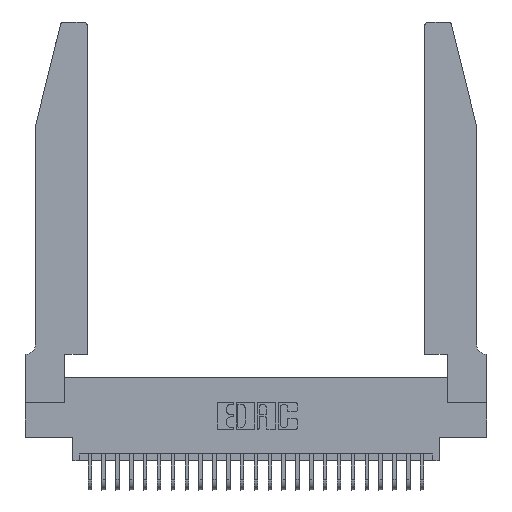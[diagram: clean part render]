
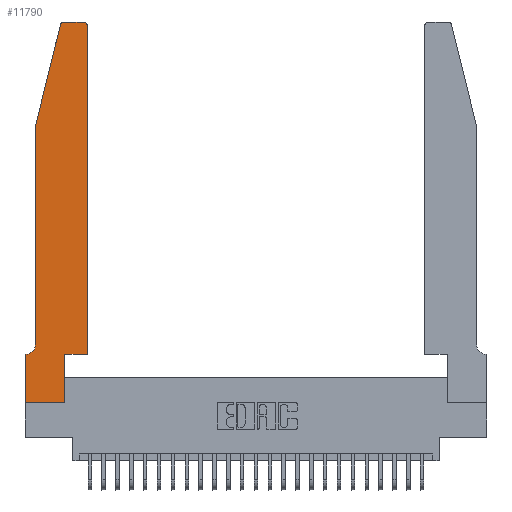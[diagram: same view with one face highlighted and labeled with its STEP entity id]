
A CAD part, top view. The second image highlights one B-rep face of the part: STEP entity #11790.
In plain terms, the highlighted planar face has unit normal (0, 0, 1).
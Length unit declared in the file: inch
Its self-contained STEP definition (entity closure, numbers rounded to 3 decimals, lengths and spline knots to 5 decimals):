
#245 = LINE ( 'NONE', #523, #20498 ) ;
#523 = CARTESIAN_POINT ( 'NONE',  ( 0.0755, 0.35, 0.37 ) ) ;
#1278 = ORIENTED_EDGE ( 'NONE', *, *, #17317, .T. ) ;
#1521 = AXIS2_PLACEMENT_3D ( 'NONE', #6994, #6895, #2677 ) ;
#1641 = CIRCLE ( 'NONE', #21112, 0.03 ) ;
#1778 = EDGE_CURVE ( 'NONE', #19641, #9027, #1641, .T. ) ;
#1780 = CARTESIAN_POINT ( 'NONE',  ( 0.2865, 0.35, 0.37 ) ) ;
#1938 = DIRECTION ( 'NONE',  ( 1., 0., 0. ) ) ;
#2074 = CARTESIAN_POINT ( 'NONE',  ( 0.284, 2.72, 0.37 ) ) ;
#2219 = FACE_OUTER_BOUND ( 'NONE', #3874, .T. ) ;
#2499 = EDGE_CURVE ( 'NONE', #19271, #24908, #20845, .T. ) ;
#2677 = DIRECTION ( 'NONE',  ( 1., 0., 0. ) ) ;
#2986 = CARTESIAN_POINT ( 'NONE',  ( 0., 0., 0.37 ) ) ;
#3343 = CARTESIAN_POINT ( 'NONE',  ( 0.0755, 2., 0.37 ) ) ;
#3530 = CARTESIAN_POINT ( 'NONE',  ( 0.4505, 0.35, 0.37 ) ) ;
#3630 = ORIENTED_EDGE ( 'NONE', *, *, #6180, .T. ) ;
#3775 = CARTESIAN_POINT ( 'NONE',  ( 0.4505, 0.35, 0.37 ) ) ;
#3874 = EDGE_LOOP ( 'NONE', ( #24590, #8716, #17306, #4096, #16593, #4768, #3630, #4051, #1278, #9621, #7478, #21929 ) ) ;
#3990 = LINE ( 'NONE', #16362, #8778 ) ;
#4051 = ORIENTED_EDGE ( 'NONE', *, *, #5038, .T. ) ;
#4096 = ORIENTED_EDGE ( 'NONE', *, *, #2499, .T. ) ;
#4520 = PLANE ( 'NONE',  #1521 ) ;
#4768 = ORIENTED_EDGE ( 'NONE', *, *, #10371, .T. ) ;
#5028 = CARTESIAN_POINT ( 'NONE',  ( 0.0755, 2., 0.37 ) ) ;
#5038 = EDGE_CURVE ( 'NONE', #8601, #7499, #10702, .T. ) ;
#5151 = DIRECTION ( 'NONE',  ( -1., 0., 0. ) ) ;
#5247 = CIRCLE ( 'NONE', #26849, 0.03 ) ;
#5271 = VECTOR ( 'NONE', #9316, 39.37008 ) ;
#6180 = EDGE_CURVE ( 'NONE', #15876, #8601, #17495, .T. ) ;
#6843 = VECTOR ( 'NONE', #8771, 39.37008 ) ;
#6895 = DIRECTION ( 'NONE',  ( 0., 0., 1. ) ) ;
#6994 = CARTESIAN_POINT ( 'NONE',  ( 0., 0.35, 0.37 ) ) ;
#7065 = LINE ( 'NONE', #3530, #20458 ) ;
#7282 = DIRECTION ( 'NONE',  ( 1., 0., 0. ) ) ;
#7478 = ORIENTED_EDGE ( 'NONE', *, *, #26118, .T. ) ;
#7499 = VERTEX_POINT ( 'NONE', #27131 ) ;
#8466 = VECTOR ( 'NONE', #15667, 39.37008 ) ;
#8601 = VERTEX_POINT ( 'NONE', #2986 ) ;
#8693 = LINE ( 'NONE', #5028, #5271 ) ;
#8716 = ORIENTED_EDGE ( 'NONE', *, *, #1778, .T. ) ;
#8771 = DIRECTION ( 'NONE',  ( 0., -1., 0. ) ) ;
#8778 = VECTOR ( 'NONE', #7282, 39.37008 ) ;
#8889 = VECTOR ( 'NONE', #5151, 39.37008 ) ;
#8951 = DIRECTION ( 'NONE',  ( 1., 0., 0. ) ) ;
#9027 = VERTEX_POINT ( 'NONE', #12243 ) ;
#9111 = CARTESIAN_POINT ( 'NONE',  ( 0.0055, 0.35, 0.37 ) ) ;
#9316 = DIRECTION ( 'NONE',  ( -0.239, -0.971, 0. ) ) ;
#9425 = VERTEX_POINT ( 'NONE', #1780 ) ;
#9621 = ORIENTED_EDGE ( 'NONE', *, *, #10871, .T. ) ;
#9690 = LINE ( 'NONE', #15055, #12479 ) ;
#9885 = VERTEX_POINT ( 'NONE', #12003 ) ;
#10371 = EDGE_CURVE ( 'NONE', #27764, #15876, #245, .T. ) ;
#10641 = DIRECTION ( 'NONE',  ( 0., 1., 0. ) ) ;
#10702 = LINE ( 'NONE', #23131, #15514 ) ;
#10871 = EDGE_CURVE ( 'NONE', #9425, #25002, #3990, .T. ) ;
#10934 = DIRECTION ( 'NONE',  ( 0., 0., 1. ) ) ;
#11790 = ADVANCED_FACE ( 'NONE', ( #2219 ), #4520, .T. ) ;
#12003 = CARTESIAN_POINT ( 'NONE',  ( 0.4205, 2.75, 0.37 ) ) ;
#12243 = CARTESIAN_POINT ( 'NONE',  ( 0.25487, 2.72718, 0.37 ) ) ;
#12479 = VECTOR ( 'NONE', #10641, 39.37008 ) ;
#13071 = CARTESIAN_POINT ( 'NONE',  ( 0.4205, 2.72, 0.37 ) ) ;
#13493 = CARTESIAN_POINT ( 'NONE',  ( 0.0755, 2., 0.37 ) ) ;
#13542 = AXIS2_PLACEMENT_3D ( 'NONE', #13786, #13961, #27164 ) ;
#13703 = LINE ( 'NONE', #26976, #8889 ) ;
#13786 = CARTESIAN_POINT ( 'NONE',  ( 0.0055, 0.42, 0.37 ) ) ;
#13884 = CARTESIAN_POINT ( 'NONE',  ( 0.284, 2.75, 0.37 ) ) ;
#13961 = DIRECTION ( 'NONE',  ( 0., 0., -1. ) ) ;
#14695 = CARTESIAN_POINT ( 'NONE',  ( 0.0755, 0.42, 0.37 ) ) ;
#15055 = CARTESIAN_POINT ( 'NONE',  ( 0.2865, 0.35, 0.37 ) ) ;
#15292 = DIRECTION ( 'NONE',  ( 0., 0., 1. ) ) ;
#15514 = VECTOR ( 'NONE', #26990, 39.37008 ) ;
#15667 = DIRECTION ( 'NONE',  ( 0., -1., 0. ) ) ;
#15876 = VERTEX_POINT ( 'NONE', #21928 ) ;
#16019 = DIRECTION ( 'NONE',  ( -1., 0., 0. ) ) ;
#16362 = CARTESIAN_POINT ( 'NONE',  ( 0.4505, 0.35, 0.37 ) ) ;
#16593 = ORIENTED_EDGE ( 'NONE', *, *, #26549, .T. ) ;
#16851 = DIRECTION ( 'NONE',  ( 0., 1., 0. ) ) ;
#17018 = EDGE_CURVE ( 'NONE', #9027, #19271, #8693, .T. ) ;
#17306 = ORIENTED_EDGE ( 'NONE', *, *, #17018, .T. ) ;
#17317 = EDGE_CURVE ( 'NONE', #7499, #9425, #9690, .T. ) ;
#17323 = EDGE_CURVE ( 'NONE', #27367, #9885, #5247, .T. ) ;
#17495 = LINE ( 'NONE', #26754, #6843 ) ;
#19271 = VERTEX_POINT ( 'NONE', #3343 ) ;
#19401 = CIRCLE ( 'NONE', #13542, 0.07 ) ;
#19409 = CARTESIAN_POINT ( 'NONE',  ( 0.4505, 2.72, 0.37 ) ) ;
#19641 = VERTEX_POINT ( 'NONE', #13884 ) ;
#19714 = EDGE_CURVE ( 'NONE', #9885, #19641, #13703, .T. ) ;
#20458 = VECTOR ( 'NONE', #16851, 39.37008 ) ;
#20498 = VECTOR ( 'NONE', #16019, 39.37008 ) ;
#20845 = LINE ( 'NONE', #13493, #8466 ) ;
#21112 = AXIS2_PLACEMENT_3D ( 'NONE', #2074, #15292, #8951 ) ;
#21928 = CARTESIAN_POINT ( 'NONE',  ( 0., 0.35, 0.37 ) ) ;
#21929 = ORIENTED_EDGE ( 'NONE', *, *, #17323, .T. ) ;
#23131 = CARTESIAN_POINT ( 'NONE',  ( 0., 0., 0.37 ) ) ;
#24590 = ORIENTED_EDGE ( 'NONE', *, *, #19714, .T. ) ;
#24908 = VERTEX_POINT ( 'NONE', #14695 ) ;
#25002 = VERTEX_POINT ( 'NONE', #3775 ) ;
#26118 = EDGE_CURVE ( 'NONE', #25002, #27367, #7065, .T. ) ;
#26549 = EDGE_CURVE ( 'NONE', #24908, #27764, #19401, .T. ) ;
#26754 = CARTESIAN_POINT ( 'NONE',  ( 0., 0., 0.37 ) ) ;
#26849 = AXIS2_PLACEMENT_3D ( 'NONE', #13071, #10934, #1938 ) ;
#26976 = CARTESIAN_POINT ( 'NONE',  ( 0.2605, 2.75, 0.37 ) ) ;
#26990 = DIRECTION ( 'NONE',  ( 1., 0., 0. ) ) ;
#27131 = CARTESIAN_POINT ( 'NONE',  ( 0.2865, 0., 0.37 ) ) ;
#27164 = DIRECTION ( 'NONE',  ( -1., 0., 0. ) ) ;
#27367 = VERTEX_POINT ( 'NONE', #19409 ) ;
#27764 = VERTEX_POINT ( 'NONE', #9111 ) ;
